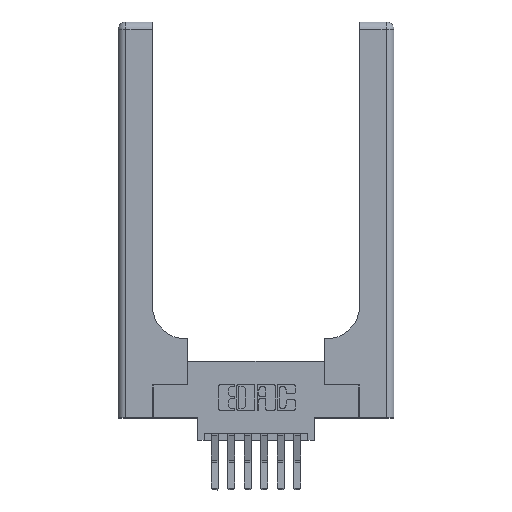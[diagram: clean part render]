
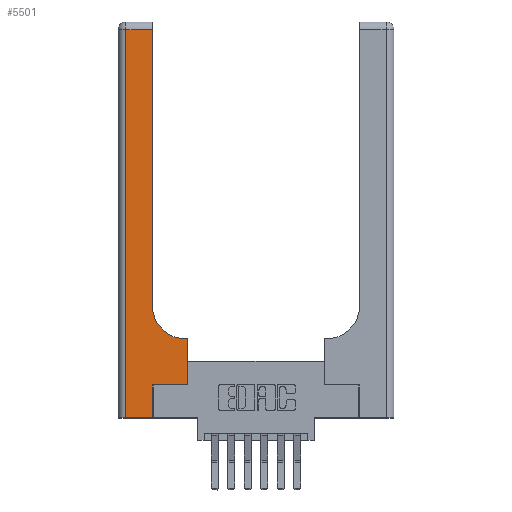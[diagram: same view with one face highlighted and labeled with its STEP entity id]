
A CAD part, top view. The second image highlights one B-rep face of the part: STEP entity #5501.
In plain terms, the highlighted planar face has unit normal (0, 0, 1).
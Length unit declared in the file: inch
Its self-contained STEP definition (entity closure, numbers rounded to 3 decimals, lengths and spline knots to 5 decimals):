
#129 = CARTESIAN_POINT ( 'NONE',  ( 0.265, 0.25, 0.37 ) ) ;
#376 = LINE ( 'NONE', #380, #6172 ) ;
#380 = CARTESIAN_POINT ( 'NONE',  ( 0.26, 0.6, 0.37 ) ) ;
#504 = PLANE ( 'NONE',  #13753 ) ;
#537 = CARTESIAN_POINT ( 'NONE',  ( 0.528, 0.6, 0.37 ) ) ;
#582 = DIRECTION ( 'NONE',  ( 0., -1., 0. ) ) ;
#934 = VECTOR ( 'NONE', #6660, 39.37008 ) ;
#1406 = EDGE_CURVE ( 'NONE', #9236, #3520, #376, .T. ) ;
#1834 = ORIENTED_EDGE ( 'NONE', *, *, #12952, .T. ) ;
#2270 = CIRCLE ( 'NONE', #9589, 0.25 ) ;
#2324 = VERTEX_POINT ( 'NONE', #9435 ) ;
#2607 = DIRECTION ( 'NONE',  ( -1., 0., 0. ) ) ;
#2751 = EDGE_CURVE ( 'NONE', #3520, #11171, #2270, .T. ) ;
#2849 = VECTOR ( 'NONE', #582, 39.37008 ) ;
#3044 = ORIENTED_EDGE ( 'NONE', *, *, #8894, .T. ) ;
#3058 = DIRECTION ( 'NONE',  ( 1., 0., 0. ) ) ;
#3115 = VECTOR ( 'NONE', #9151, 39.37008 ) ;
#3185 = LINE ( 'NONE', #12545, #2849 ) ;
#3300 = VERTEX_POINT ( 'NONE', #13098 ) ;
#3421 = EDGE_CURVE ( 'NONE', #2324, #9236, #5970, .T. ) ;
#3520 = VERTEX_POINT ( 'NONE', #9389 ) ;
#3591 = ORIENTED_EDGE ( 'NONE', *, *, #12534, .T. ) ;
#3601 = CARTESIAN_POINT ( 'NONE',  ( 0.06, 2.94, 0.37 ) ) ;
#4493 = ORIENTED_EDGE ( 'NONE', *, *, #8870, .T. ) ;
#4542 = VERTEX_POINT ( 'NONE', #3601 ) ;
#4591 = ORIENTED_EDGE ( 'NONE', *, *, #3421, .T. ) ;
#4905 = DIRECTION ( 'NONE',  ( 0., 0., -1. ) ) ;
#5032 = CARTESIAN_POINT ( 'NONE',  ( 0.265, 0., 0.37 ) ) ;
#5123 = VECTOR ( 'NONE', #3058, 39.37008 ) ;
#5149 = VECTOR ( 'NONE', #9226, 39.37008 ) ;
#5354 = CARTESIAN_POINT ( 'NONE',  ( 0.26, 2.94, 0.37 ) ) ;
#5501 = ADVANCED_FACE ( 'NONE', ( #7926 ), #504, .F. ) ;
#5545 = VERTEX_POINT ( 'NONE', #8190 ) ;
#5669 = CARTESIAN_POINT ( 'NONE',  ( 0.51, 0.85, 0.37 ) ) ;
#5788 = DIRECTION ( 'NONE',  ( -1., 0., 0. ) ) ;
#5918 = EDGE_LOOP ( 'NONE', ( #3044, #12464, #3591, #4493, #11747, #1834, #4591, #14005, #13214 ) ) ;
#5970 = LINE ( 'NONE', #12439, #3115 ) ;
#6172 = VECTOR ( 'NONE', #2607, 39.37008 ) ;
#6660 = DIRECTION ( 'NONE',  ( 1., 0., 0. ) ) ;
#6763 = DIRECTION ( 'NONE',  ( 1., 0., 0. ) ) ;
#7059 = LINE ( 'NONE', #129, #934 ) ;
#7111 = CARTESIAN_POINT ( 'NONE',  ( 0.26, 0.85, 0.37 ) ) ;
#7408 = CARTESIAN_POINT ( 'NONE',  ( 0.26, 3., 0.37 ) ) ;
#7667 = LINE ( 'NONE', #7408, #13166 ) ;
#7799 = EDGE_CURVE ( 'NONE', #3300, #5545, #10958, .T. ) ;
#7926 = FACE_OUTER_BOUND ( 'NONE', #5918, .T. ) ;
#7945 = CARTESIAN_POINT ( 'NONE',  ( 0., 2.94, 0.37 ) ) ;
#8010 = LINE ( 'NONE', #9568, #5123 ) ;
#8175 = VECTOR ( 'NONE', #5788, 39.37008 ) ;
#8190 = CARTESIAN_POINT ( 'NONE',  ( 0.265, 0.25, 0.37 ) ) ;
#8508 = DIRECTION ( 'NONE',  ( 0., 1., 0. ) ) ;
#8870 = EDGE_CURVE ( 'NONE', #9704, #3300, #8010, .T. ) ;
#8894 = EDGE_CURVE ( 'NONE', #11171, #12238, #7667, .T. ) ;
#9005 = CARTESIAN_POINT ( 'NONE',  ( 0.06, 0., 0.37 ) ) ;
#9151 = DIRECTION ( 'NONE',  ( 0., 1., 0. ) ) ;
#9226 = DIRECTION ( 'NONE',  ( 0., 1., 0. ) ) ;
#9236 = VERTEX_POINT ( 'NONE', #537 ) ;
#9389 = CARTESIAN_POINT ( 'NONE',  ( 0.51, 0.6, 0.37 ) ) ;
#9435 = CARTESIAN_POINT ( 'NONE',  ( 0.528, 0.25, 0.37 ) ) ;
#9568 = CARTESIAN_POINT ( 'NONE',  ( 0., 0., 0.37 ) ) ;
#9589 = AXIS2_PLACEMENT_3D ( 'NONE', #5669, #13341, #6763 ) ;
#9704 = VERTEX_POINT ( 'NONE', #9005 ) ;
#10323 = EDGE_CURVE ( 'NONE', #12238, #4542, #11085, .T. ) ;
#10958 = LINE ( 'NONE', #5032, #5149 ) ;
#11085 = LINE ( 'NONE', #7945, #8175 ) ;
#11171 = VERTEX_POINT ( 'NONE', #7111 ) ;
#11359 = CARTESIAN_POINT ( 'NONE',  ( 0., 3., 0.37 ) ) ;
#11747 = ORIENTED_EDGE ( 'NONE', *, *, #7799, .T. ) ;
#12238 = VERTEX_POINT ( 'NONE', #5354 ) ;
#12439 = CARTESIAN_POINT ( 'NONE',  ( 0.528, 0.25, 0.37 ) ) ;
#12464 = ORIENTED_EDGE ( 'NONE', *, *, #10323, .T. ) ;
#12534 = EDGE_CURVE ( 'NONE', #4542, #9704, #3185, .T. ) ;
#12545 = CARTESIAN_POINT ( 'NONE',  ( 0.06, 3., 0.37 ) ) ;
#12567 = DIRECTION ( 'NONE',  ( -1., 0., 0. ) ) ;
#12952 = EDGE_CURVE ( 'NONE', #5545, #2324, #7059, .T. ) ;
#13098 = CARTESIAN_POINT ( 'NONE',  ( 0.265, 0., 0.37 ) ) ;
#13166 = VECTOR ( 'NONE', #8508, 39.37008 ) ;
#13214 = ORIENTED_EDGE ( 'NONE', *, *, #2751, .T. ) ;
#13341 = DIRECTION ( 'NONE',  ( 0., 0., -1. ) ) ;
#13753 = AXIS2_PLACEMENT_3D ( 'NONE', #11359, #4905, #12567 ) ;
#14005 = ORIENTED_EDGE ( 'NONE', *, *, #1406, .T. ) ;
